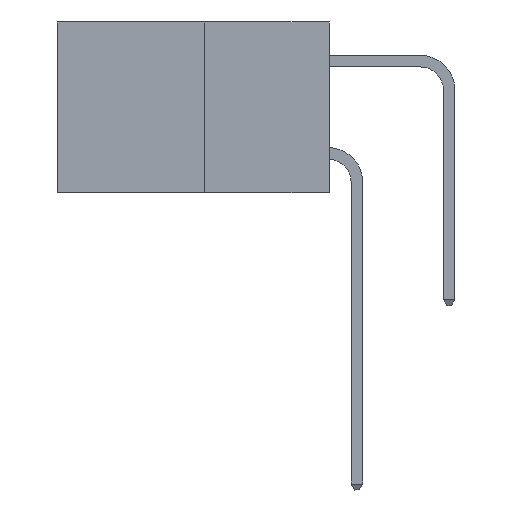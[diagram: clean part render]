
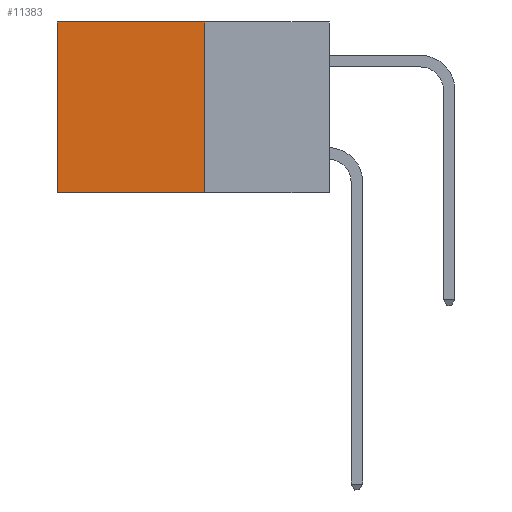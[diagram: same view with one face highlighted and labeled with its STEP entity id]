
A CAD part, left-side view. The second image highlights one B-rep face of the part: STEP entity #11383.
In plain terms, the highlighted planar face has unit normal (-1, 0, 0).
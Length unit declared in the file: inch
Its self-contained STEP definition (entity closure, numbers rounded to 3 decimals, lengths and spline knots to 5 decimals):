
#20 = EDGE_CURVE ( 'NONE', #12117, #24819, #18484, .T. ) ;
#269 = ORIENTED_EDGE ( 'NONE', *, *, #20, .F. ) ;
#1055 = EDGE_CURVE ( 'NONE', #24819, #10581, #9983, .T. ) ;
#1385 = ORIENTED_EDGE ( 'NONE', *, *, #1055, .F. ) ;
#2399 = FACE_OUTER_BOUND ( 'NONE', #15560, .T. ) ;
#2668 = DIRECTION ( 'NONE',  ( 1., 0., 0. ) ) ;
#4052 = VECTOR ( 'NONE', #21321, 39.37008 ) ;
#5761 = CARTESIAN_POINT ( 'NONE',  ( 0.277, 0.27, -0.37 ) ) ;
#5783 = ORIENTED_EDGE ( 'NONE', *, *, #10610, .T. ) ;
#6624 = CARTESIAN_POINT ( 'NONE',  ( 0.277, 0.27, -0.37 ) ) ;
#7722 = AXIS2_PLACEMENT_3D ( 'NONE', #23347, #2668, #17234 ) ;
#8653 = CARTESIAN_POINT ( 'NONE',  ( 0.277, 0.59, -0.37 ) ) ;
#8973 = CARTESIAN_POINT ( 'NONE',  ( 0.277, 0.59, 0. ) ) ;
#9416 = ORIENTED_EDGE ( 'NONE', *, *, #20797, .T. ) ;
#9983 = LINE ( 'NONE', #6624, #20365 ) ;
#10285 = VECTOR ( 'NONE', #23109, 39.37008 ) ;
#10581 = VERTEX_POINT ( 'NONE', #10634 ) ;
#10610 = EDGE_CURVE ( 'NONE', #26569, #10581, #26683, .T. ) ;
#10634 = CARTESIAN_POINT ( 'NONE',  ( 0.277, 0.59, -0.37 ) ) ;
#11383 = ADVANCED_FACE ( 'NONE', ( #2399 ), #15116, .F. ) ;
#12117 = VERTEX_POINT ( 'NONE', #26696 ) ;
#13612 = VECTOR ( 'NONE', #24735, 39.37008 ) ;
#15116 = PLANE ( 'NONE',  #7722 ) ;
#15560 = EDGE_LOOP ( 'NONE', ( #5783, #1385, #269, #9416 ) ) ;
#17234 = DIRECTION ( 'NONE',  ( 0., 0., -1. ) ) ;
#18484 = LINE ( 'NONE', #25653, #13612 ) ;
#19266 = CARTESIAN_POINT ( 'NONE',  ( 0.277, 0.27, 0. ) ) ;
#20365 = VECTOR ( 'NONE', #22603, 39.37008 ) ;
#20797 = EDGE_CURVE ( 'NONE', #12117, #26569, #26024, .T. ) ;
#21321 = DIRECTION ( 'NONE',  ( 0., 1., 0. ) ) ;
#22603 = DIRECTION ( 'NONE',  ( 0., 1., 0. ) ) ;
#23109 = DIRECTION ( 'NONE',  ( 0., 0., -1. ) ) ;
#23347 = CARTESIAN_POINT ( 'NONE',  ( 0.277, 0.27, -0.37 ) ) ;
#24735 = DIRECTION ( 'NONE',  ( 0., 0., -1. ) ) ;
#24819 = VERTEX_POINT ( 'NONE', #5761 ) ;
#25653 = CARTESIAN_POINT ( 'NONE',  ( 0.277, 0.27, -0.37 ) ) ;
#26024 = LINE ( 'NONE', #19266, #4052 ) ;
#26569 = VERTEX_POINT ( 'NONE', #8973 ) ;
#26683 = LINE ( 'NONE', #8653, #10285 ) ;
#26696 = CARTESIAN_POINT ( 'NONE',  ( 0.277, 0.27, 0. ) ) ;
